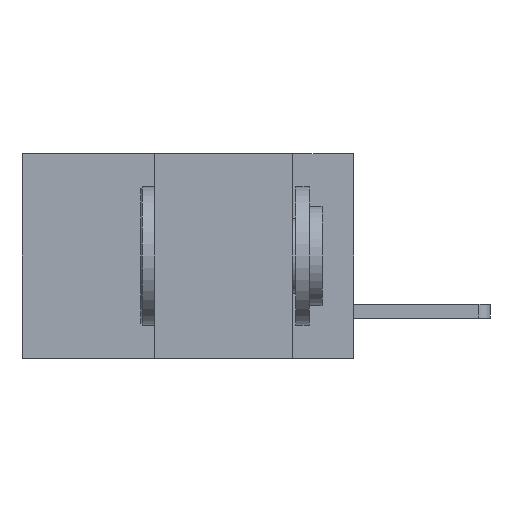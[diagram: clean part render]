
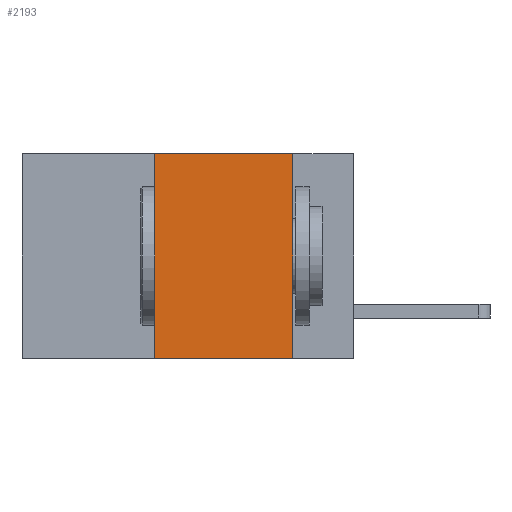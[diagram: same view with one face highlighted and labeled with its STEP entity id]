
A CAD part, left-side view. The second image highlights one B-rep face of the part: STEP entity #2193.
In plain terms, the highlighted planar face has unit normal (-1, 0, 0).
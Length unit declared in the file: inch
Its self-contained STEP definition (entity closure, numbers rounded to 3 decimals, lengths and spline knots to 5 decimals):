
#20 = AXIS2_PLACEMENT_3D ( 'NONE', #1172, #1834, #8968 ) ;
#543 = CARTESIAN_POINT ( 'NONE',  ( 0., 0.6, 0. ) ) ;
#588 = VECTOR ( 'NONE', #7505, 39.37008 ) ;
#929 = LINE ( 'NONE', #8919, #4807 ) ;
#989 = CARTESIAN_POINT ( 'NONE',  ( 0., 0.6, -0.37 ) ) ;
#991 = VECTOR ( 'NONE', #6690, 39.37008 ) ;
#1172 = CARTESIAN_POINT ( 'NONE',  ( 0., 0.6, 0. ) ) ;
#1592 = VERTEX_POINT ( 'NONE', #5404 ) ;
#1834 = DIRECTION ( 'NONE',  ( 1., 0., 0. ) ) ;
#2193 = ADVANCED_FACE ( 'NONE', ( #4080 ), #9062, .F. ) ;
#3170 = ORIENTED_EDGE ( 'NONE', *, *, #6005, .T. ) ;
#3474 = DIRECTION ( 'NONE',  ( 0., -1., 0. ) ) ;
#3818 = CARTESIAN_POINT ( 'NONE',  ( 0., 0.36, 0. ) ) ;
#3998 = ORIENTED_EDGE ( 'NONE', *, *, #5182, .F. ) ;
#4027 = LINE ( 'NONE', #543, #9228 ) ;
#4080 = FACE_OUTER_BOUND ( 'NONE', #5484, .T. ) ;
#4423 = DIRECTION ( 'NONE',  ( 0., 0., -1. ) ) ;
#4586 = LINE ( 'NONE', #6698, #588 ) ;
#4807 = VECTOR ( 'NONE', #4423, 39.37008 ) ;
#4884 = CARTESIAN_POINT ( 'NONE',  ( 0., 0.11, -0.37 ) ) ;
#5138 = ORIENTED_EDGE ( 'NONE', *, *, #7531, .F. ) ;
#5182 = EDGE_CURVE ( 'NONE', #9348, #8587, #4027, .T. ) ;
#5404 = CARTESIAN_POINT ( 'NONE',  ( 0., 0.36, -0.37 ) ) ;
#5484 = EDGE_LOOP ( 'NONE', ( #7274, #3998, #5138, #3170 ) ) ;
#5523 = VERTEX_POINT ( 'NONE', #4884 ) ;
#6005 = EDGE_CURVE ( 'NONE', #1592, #5523, #6839, .T. ) ;
#6690 = DIRECTION ( 'NONE',  ( 0., -1., 0. ) ) ;
#6698 = CARTESIAN_POINT ( 'NONE',  ( 0., 0.36, 0. ) ) ;
#6839 = LINE ( 'NONE', #989, #991 ) ;
#7110 = CARTESIAN_POINT ( 'NONE',  ( 0., 0.11, 0. ) ) ;
#7274 = ORIENTED_EDGE ( 'NONE', *, *, #8351, .F. ) ;
#7505 = DIRECTION ( 'NONE',  ( 0., 0., 1. ) ) ;
#7531 = EDGE_CURVE ( 'NONE', #1592, #9348, #4586, .T. ) ;
#8351 = EDGE_CURVE ( 'NONE', #8587, #5523, #929, .T. ) ;
#8587 = VERTEX_POINT ( 'NONE', #7110 ) ;
#8919 = CARTESIAN_POINT ( 'NONE',  ( 0., 0.11, 0. ) ) ;
#8968 = DIRECTION ( 'NONE',  ( 0., 0., -1. ) ) ;
#9062 = PLANE ( 'NONE',  #20 ) ;
#9228 = VECTOR ( 'NONE', #3474, 39.37008 ) ;
#9348 = VERTEX_POINT ( 'NONE', #3818 ) ;
